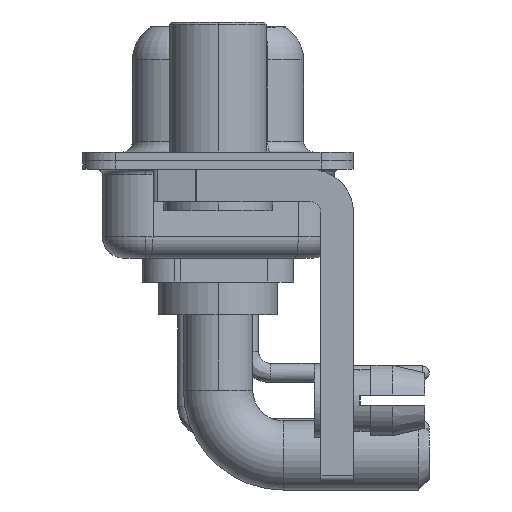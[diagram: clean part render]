
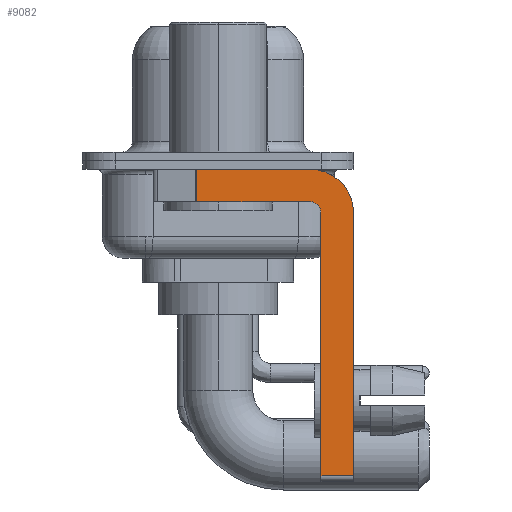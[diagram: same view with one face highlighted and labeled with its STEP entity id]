
A CAD part, left-side view. The second image highlights one B-rep face of the part: STEP entity #9082.
In plain terms, the highlighted planar face has unit normal (-1, 0, 0).
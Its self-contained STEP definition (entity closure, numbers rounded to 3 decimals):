
#755 = VECTOR ( 'NONE', #21693, 1000. ) ;
#812 = VECTOR ( 'NONE', #3202, 1000. ) ;
#844 = ORIENTED_EDGE ( 'NONE', *, *, #8597, .F. ) ;
#1080 = ORIENTED_EDGE ( 'NONE', *, *, #11903, .F. ) ;
#1396 = AXIS2_PLACEMENT_3D ( 'NONE', #23420, #8296, #12961 ) ;
#1556 = EDGE_LOOP ( 'NONE', ( #20578, #8703, #1080, #17699, #5125, #14468, #844, #23289 ) ) ;
#2662 = DIRECTION ( 'NONE',  ( 0., 1., 0. ) ) ;
#2957 = VERTEX_POINT ( 'NONE', #24090 ) ;
#3060 = CARTESIAN_POINT ( 'NONE',  ( -2.9, 3., -0.4 ) ) ;
#3202 = DIRECTION ( 'NONE',  ( 0., -1., 0. ) ) ;
#4066 = CARTESIAN_POINT ( 'NONE',  ( -2.9, -6.25, -2.4 ) ) ;
#4328 = CARTESIAN_POINT ( 'NONE',  ( -2.9, -4.25, -1.9 ) ) ;
#5125 = ORIENTED_EDGE ( 'NONE', *, *, #26909, .F. ) ;
#5174 = CARTESIAN_POINT ( 'NONE',  ( -2.9, 0.978, -1.9 ) ) ;
#6837 = LINE ( 'NONE', #5174, #755 ) ;
#7257 = CARTESIAN_POINT ( 'NONE',  ( -2.9, -4.75, -14.55 ) ) ;
#7280 = DIRECTION ( 'NONE',  ( 0., 0., 1. ) ) ;
#7393 = CARTESIAN_POINT ( 'NONE',  ( -2.9, -4.25, -0.4 ) ) ;
#8173 = CARTESIAN_POINT ( 'NONE',  ( -2.9, -4.75, -14.8 ) ) ;
#8296 = DIRECTION ( 'NONE',  ( 1., 0., 0. ) ) ;
#8321 = VERTEX_POINT ( 'NONE', #24154 ) ;
#8597 = EDGE_CURVE ( 'NONE', #8321, #2957, #23043, .T. ) ;
#8703 = ORIENTED_EDGE ( 'NONE', *, *, #12889, .T. ) ;
#8746 = VERTEX_POINT ( 'NONE', #13544 ) ;
#9082 = ADVANCED_FACE ( 'NONE', ( #12956 ), #15068, .F. ) ;
#9635 = CIRCLE ( 'NONE', #12711, 0.5 ) ;
#11275 = CARTESIAN_POINT ( 'NONE',  ( -2.9, -4.25, -2.4 ) ) ;
#11459 = CARTESIAN_POINT ( 'NONE',  ( -2.9, 0.978, -1.9 ) ) ;
#11588 = VECTOR ( 'NONE', #14281, 1000. ) ;
#11903 = EDGE_CURVE ( 'NONE', #8746, #19377, #21648, .T. ) ;
#12711 = AXIS2_PLACEMENT_3D ( 'NONE', #11275, #17984, #7280 ) ;
#12889 = EDGE_CURVE ( 'NONE', #13236, #19377, #6837, .T. ) ;
#12956 = FACE_OUTER_BOUND ( 'NONE', #1556, .T. ) ;
#12961 = DIRECTION ( 'NONE',  ( 0., 0., -1. ) ) ;
#13236 = VERTEX_POINT ( 'NONE', #21933 ) ;
#13544 = CARTESIAN_POINT ( 'NONE',  ( -2.9, -4.25, -1.9 ) ) ;
#13905 = EDGE_CURVE ( 'NONE', #13236, #18810, #15655, .T. ) ;
#14281 = DIRECTION ( 'NONE',  ( 0., 0., 1. ) ) ;
#14311 = EDGE_CURVE ( 'NONE', #14692, #8746, #9635, .T. ) ;
#14468 = ORIENTED_EDGE ( 'NONE', *, *, #17762, .T. ) ;
#14692 = VERTEX_POINT ( 'NONE', #26540 ) ;
#14703 = DIRECTION ( 'NONE',  ( 0., 0., -1. ) ) ;
#14779 = AXIS2_PLACEMENT_3D ( 'NONE', #17157, #19246, #23682 ) ;
#15068 = PLANE ( 'NONE',  #14779 ) ;
#15383 = DIRECTION ( 'NONE',  ( 0., -1., 0. ) ) ;
#15655 = LINE ( 'NONE', #3060, #812 ) ;
#16955 = EDGE_CURVE ( 'NONE', #18810, #8321, #25274, .T. ) ;
#17157 = CARTESIAN_POINT ( 'NONE',  ( -2.9, -4.25, -2.4 ) ) ;
#17699 = ORIENTED_EDGE ( 'NONE', *, *, #14311, .F. ) ;
#17762 = EDGE_CURVE ( 'NONE', #24403, #2957, #21647, .T. ) ;
#17984 = DIRECTION ( 'NONE',  ( -1., 0., 0. ) ) ;
#18810 = VERTEX_POINT ( 'NONE', #7393 ) ;
#19246 = DIRECTION ( 'NONE',  ( 1., 0., 0. ) ) ;
#19377 = VERTEX_POINT ( 'NONE', #11459 ) ;
#19423 = VECTOR ( 'NONE', #14703, 1000. ) ;
#20578 = ORIENTED_EDGE ( 'NONE', *, *, #13905, .F. ) ;
#20624 = VECTOR ( 'NONE', #2662, 1000. ) ;
#21647 = LINE ( 'NONE', #23588, #24801 ) ;
#21648 = LINE ( 'NONE', #4328, #20624 ) ;
#21693 = DIRECTION ( 'NONE',  ( 0., 0., -1. ) ) ;
#21933 = CARTESIAN_POINT ( 'NONE',  ( -2.9, 0.978, -0.4 ) ) ;
#23043 = LINE ( 'NONE', #4066, #19423 ) ;
#23289 = ORIENTED_EDGE ( 'NONE', *, *, #16955, .F. ) ;
#23420 = CARTESIAN_POINT ( 'NONE',  ( -2.9, -4.25, -2.4 ) ) ;
#23588 = CARTESIAN_POINT ( 'NONE',  ( -2.9, -4.25, -14.55 ) ) ;
#23682 = DIRECTION ( 'NONE',  ( 0., 0., -1. ) ) ;
#24090 = CARTESIAN_POINT ( 'NONE',  ( -2.9, -6.25, -14.55 ) ) ;
#24154 = CARTESIAN_POINT ( 'NONE',  ( -2.9, -6.25, -2.4 ) ) ;
#24403 = VERTEX_POINT ( 'NONE', #7257 ) ;
#24801 = VECTOR ( 'NONE', #15383, 1000. ) ;
#25274 = CIRCLE ( 'NONE', #1396, 2. ) ;
#26540 = CARTESIAN_POINT ( 'NONE',  ( -2.9, -4.75, -2.4 ) ) ;
#26777 = LINE ( 'NONE', #8173, #11588 ) ;
#26909 = EDGE_CURVE ( 'NONE', #24403, #14692, #26777, .T. ) ;
